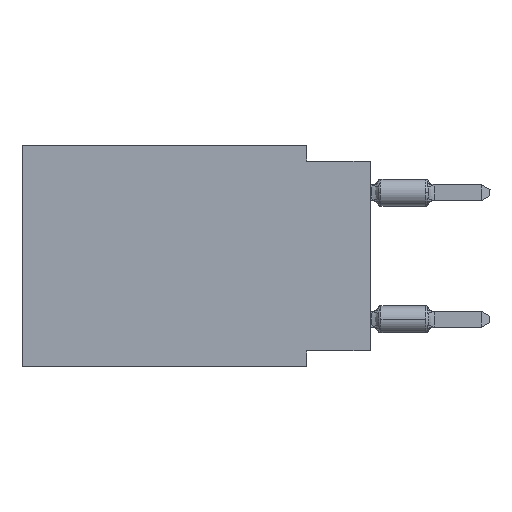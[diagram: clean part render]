
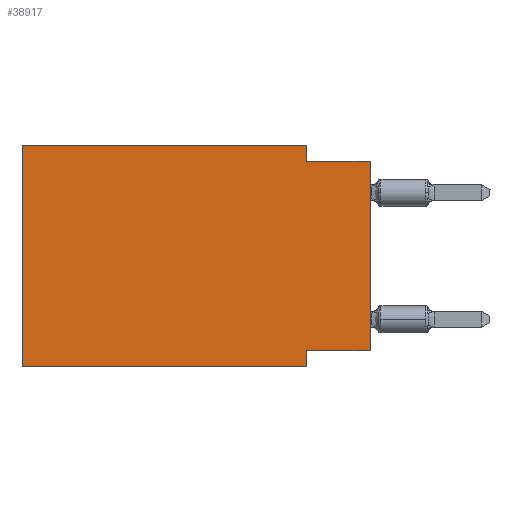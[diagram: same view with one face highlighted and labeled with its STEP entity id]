
A CAD part, left-side view. The second image highlights one B-rep face of the part: STEP entity #38917.
In plain terms, the highlighted planar face has unit normal (-1, 0, 0).
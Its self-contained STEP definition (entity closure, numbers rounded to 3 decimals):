
#565 = VECTOR ( 'NONE', #25386, 1000. ) ;
#1588 = DIRECTION ( 'NONE',  ( 0., 1., 0. ) ) ;
#2019 = AXIS2_PLACEMENT_3D ( 'NONE', #4410, #59398, #26492 ) ;
#3049 = LINE ( 'NONE', #16341, #41093 ) ;
#4410 = CARTESIAN_POINT ( 'NONE',  ( 0., 13.97, 0. ) ) ;
#4609 = ORIENTED_EDGE ( 'NONE', *, *, #50057, .T. ) ;
#5378 = VERTEX_POINT ( 'NONE', #42105 ) ;
#5627 = EDGE_CURVE ( 'NONE', #16333, #12941, #40553, .T. ) ;
#6091 = EDGE_LOOP ( 'NONE', ( #4609, #6957, #44708, #41557, #35364, #39895, #22249, #24554 ) ) ;
#6957 = ORIENTED_EDGE ( 'NONE', *, *, #58053, .F. ) ;
#7354 = CARTESIAN_POINT ( 'NONE',  ( 0., 0., -0.635 ) ) ;
#7955 = DIRECTION ( 'NONE',  ( 0., -1., 0. ) ) ;
#8888 = CARTESIAN_POINT ( 'NONE',  ( 0., 0., -0.635 ) ) ;
#10531 = VECTOR ( 'NONE', #35814, 1000. ) ;
#12002 = EDGE_CURVE ( 'NONE', #57394, #45674, #3049, .T. ) ;
#12456 = VECTOR ( 'NONE', #49599, 1000. ) ;
#12941 = VERTEX_POINT ( 'NONE', #27081 ) ;
#16333 = VERTEX_POINT ( 'NONE', #48107 ) ;
#16341 = CARTESIAN_POINT ( 'NONE',  ( 0., 13.97, 0. ) ) ;
#16612 = LINE ( 'NONE', #26293, #565 ) ;
#17306 = DIRECTION ( 'NONE',  ( 0., -1., 0. ) ) ;
#17738 = CARTESIAN_POINT ( 'NONE',  ( 0., 0., -8.255 ) ) ;
#18148 = EDGE_CURVE ( 'NONE', #45674, #5378, #54465, .T. ) ;
#21763 = DIRECTION ( 'NONE',  ( 0., 0., 1. ) ) ;
#22249 = ORIENTED_EDGE ( 'NONE', *, *, #5627, .F. ) ;
#22319 = LINE ( 'NONE', #54644, #26960 ) ;
#22433 = CARTESIAN_POINT ( 'NONE',  ( 0., 13.97, 0. ) ) ;
#23300 = EDGE_CURVE ( 'NONE', #33508, #16333, #48440, .T. ) ;
#24554 = ORIENTED_EDGE ( 'NONE', *, *, #23300, .F. ) ;
#25386 = DIRECTION ( 'NONE',  ( 0., -1., 0. ) ) ;
#26293 = CARTESIAN_POINT ( 'NONE',  ( 0., 13.97, -8.89 ) ) ;
#26492 = DIRECTION ( 'NONE',  ( 0., 0., -1. ) ) ;
#26960 = VECTOR ( 'NONE', #50141, 1000. ) ;
#27081 = CARTESIAN_POINT ( 'NONE',  ( 0., 2.54, -8.89 ) ) ;
#32677 = VECTOR ( 'NONE', #17306, 1000. ) ;
#32916 = CARTESIAN_POINT ( 'NONE',  ( 0., 13.97, -8.89 ) ) ;
#32972 = VECTOR ( 'NONE', #7955, 1000. ) ;
#33508 = VERTEX_POINT ( 'NONE', #17738 ) ;
#34227 = EDGE_CURVE ( 'NONE', #57394, #12941, #16612, .T. ) ;
#34870 = LINE ( 'NONE', #7354, #32677 ) ;
#35364 = ORIENTED_EDGE ( 'NONE', *, *, #12002, .F. ) ;
#35814 = DIRECTION ( 'NONE',  ( 0., 0., 1. ) ) ;
#36237 = VECTOR ( 'NONE', #1588, 1000. ) ;
#38641 = LINE ( 'NONE', #49705, #10531 ) ;
#38792 = CARTESIAN_POINT ( 'NONE',  ( 0., 0., -8.255 ) ) ;
#38917 = ADVANCED_FACE ( 'NONE', ( #39839 ), #40725, .F. ) ;
#39839 = FACE_OUTER_BOUND ( 'NONE', #6091, .T. ) ;
#39895 = ORIENTED_EDGE ( 'NONE', *, *, #34227, .T. ) ;
#40553 = LINE ( 'NONE', #44484, #12456 ) ;
#40725 = PLANE ( 'NONE',  #2019 ) ;
#41093 = VECTOR ( 'NONE', #21763, 1000. ) ;
#41557 = ORIENTED_EDGE ( 'NONE', *, *, #18148, .F. ) ;
#42105 = CARTESIAN_POINT ( 'NONE',  ( 0., 2.54, 0. ) ) ;
#43220 = CARTESIAN_POINT ( 'NONE',  ( 0., 2.54, -0.635 ) ) ;
#44484 = CARTESIAN_POINT ( 'NONE',  ( 0., 2.54, -8.89 ) ) ;
#44708 = ORIENTED_EDGE ( 'NONE', *, *, #49808, .F. ) ;
#45674 = VERTEX_POINT ( 'NONE', #55693 ) ;
#46829 = VERTEX_POINT ( 'NONE', #8888 ) ;
#48107 = CARTESIAN_POINT ( 'NONE',  ( 0., 2.54, -8.255 ) ) ;
#48440 = LINE ( 'NONE', #38792, #36237 ) ;
#49599 = DIRECTION ( 'NONE',  ( 0., 0., -1. ) ) ;
#49705 = CARTESIAN_POINT ( 'NONE',  ( 0., 0., 0. ) ) ;
#49808 = EDGE_CURVE ( 'NONE', #5378, #50755, #22319, .T. ) ;
#50057 = EDGE_CURVE ( 'NONE', #33508, #46829, #38641, .T. ) ;
#50141 = DIRECTION ( 'NONE',  ( 0., 0., -1. ) ) ;
#50755 = VERTEX_POINT ( 'NONE', #43220 ) ;
#54465 = LINE ( 'NONE', #22433, #32972 ) ;
#54644 = CARTESIAN_POINT ( 'NONE',  ( 0., 2.54, 0. ) ) ;
#55693 = CARTESIAN_POINT ( 'NONE',  ( 0., 13.97, 0. ) ) ;
#57394 = VERTEX_POINT ( 'NONE', #32916 ) ;
#58053 = EDGE_CURVE ( 'NONE', #50755, #46829, #34870, .T. ) ;
#59398 = DIRECTION ( 'NONE',  ( 1., 0., 0. ) ) ;
